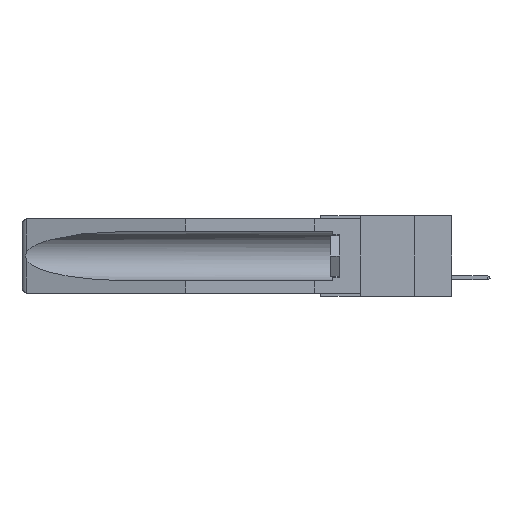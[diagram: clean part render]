
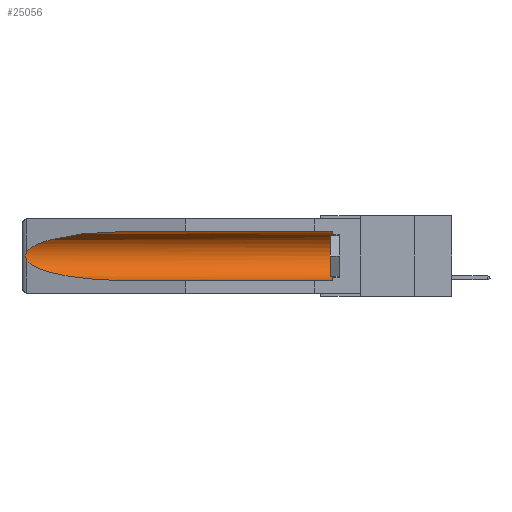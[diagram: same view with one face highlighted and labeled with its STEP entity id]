
A CAD part, left-side view. The second image highlights one B-rep face of the part: STEP entity #25056.
In plain terms, the highlighted cylindrical face has radius 2.857 mm (diameter 5.715 mm), a partial arc.
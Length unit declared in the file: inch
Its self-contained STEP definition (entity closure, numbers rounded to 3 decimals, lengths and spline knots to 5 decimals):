
#21 = CARTESIAN_POINT ( 'NONE',  ( 0.155, 1.07973, -0.284 ) ) ;
#524 = CARTESIAN_POINT ( 'NONE',  ( 0.155, 1.07973, -0.059 ) ) ;
#2341 = DIRECTION ( 'NONE',  ( 0., 1., 0. ) ) ;
#3366 = EDGE_CURVE ( 'NONE', #17460, #10818, #11243, .T. ) ;
#3832 = CIRCLE ( 'NONE', #13570, 0.1125 ) ;
#3856 =( BOUNDED_CURVE ( )  B_SPLINE_CURVE ( 3, ( #12913, #20463, #23338, #21 ),
 .UNSPECIFIED., .F., .F. ) 
 B_SPLINE_CURVE_WITH_KNOTS ( ( 4, 4 ),
 ( 0.1948, 1.5708 ),
 .UNSPECIFIED. ) 
 CURVE ( )  GEOMETRIC_REPRESENTATION_ITEM ( )  RATIONAL_B_SPLINE_CURVE ( ( 1., 0.848, 0.848, 1. ) ) 
 REPRESENTATION_ITEM ( '' )  );
#3952 = DIRECTION ( 'NONE',  ( 0., 1., 0. ) ) ;
#4195 = AXIS2_PLACEMENT_3D ( 'NONE', #27512, #2341, #12525 ) ;
#4275 = ORIENTED_EDGE ( 'NONE', *, *, #18997, .T. ) ;
#5678 = EDGE_CURVE ( 'NONE', #18760, #17460, #15857, .T. ) ;
#6527 = CARTESIAN_POINT ( 'NONE',  ( 0.26597, 1.5296, -0.19026 ) ) ;
#7708 = CARTESIAN_POINT ( 'NONE',  ( 0.26537, 1.52718, -0.19328 ) ) ;
#8341 = CARTESIAN_POINT ( 'NONE',  ( 0.2675, 1.53308, -0.17534 ) ) ;
#8485 = CARTESIAN_POINT ( 'NONE',  ( 0.21114, 1.30732, -0.059 ) ) ;
#9053 = ORIENTED_EDGE ( 'NONE', *, *, #28622, .F. ) ;
#9091 = CARTESIAN_POINT ( 'NONE',  ( 0.26655, 1.53094, -0.18657 ) ) ;
#9796 = CARTESIAN_POINT ( 'NONE',  ( 0.26597, 1.52961, -0.15275 ) ) ;
#10030 = CARTESIAN_POINT ( 'NONE',  ( 0.155, -0.30754, -0.059 ) ) ;
#10818 = VERTEX_POINT ( 'NONE', #28492 ) ;
#11243 =( BOUNDED_CURVE ( )  B_SPLINE_CURVE ( 3, ( #524, #8485, #18940, #16122 ),
 .UNSPECIFIED., .F., .F. ) 
 B_SPLINE_CURVE_WITH_KNOTS ( ( 4, 4 ),
 ( 4.71239, 6.08839 ),
 .UNSPECIFIED. ) 
 CURVE ( )  GEOMETRIC_REPRESENTATION_ITEM ( )  RATIONAL_B_SPLINE_CURVE ( ( 1., 0.848, 0.848, 1. ) ) 
 REPRESENTATION_ITEM ( '' )  );
#12525 = DIRECTION ( 'NONE',  ( 0., 0., 1. ) ) ;
#12913 = CARTESIAN_POINT ( 'NONE',  ( 0.26537, 1.52718, -0.19328 ) ) ;
#13020 = EDGE_CURVE ( 'NONE', #19597, #18760, #3832, .T. ) ;
#13570 = AXIS2_PLACEMENT_3D ( 'NONE', #16858, #19249, #19352 ) ;
#13711 = VERTEX_POINT ( 'NONE', #7708 ) ;
#14286 = VECTOR ( 'NONE', #3952, 39.37008 ) ;
#15514 = CYLINDRICAL_SURFACE ( 'NONE', #4195, 0.1125 ) ;
#15831 = ORIENTED_EDGE ( 'NONE', *, *, #3366, .T. ) ;
#15857 = LINE ( 'NONE', #10030, #21858 ) ;
#16122 = CARTESIAN_POINT ( 'NONE',  ( 0.26537, 1.52718, -0.14972 ) ) ;
#16412 = CARTESIAN_POINT ( 'NONE',  ( 0.26537, 1.52718, -0.19328 ) ) ;
#16858 = CARTESIAN_POINT ( 'NONE',  ( 0.155, 0.126, -0.1715 ) ) ;
#17098 = LINE ( 'NONE', #28050, #14286 ) ;
#17460 = VERTEX_POINT ( 'NONE', #24716 ) ;
#17918 = FACE_OUTER_BOUND ( 'NONE', #21336, .T. ) ;
#18224 = ORIENTED_EDGE ( 'NONE', *, *, #5678, .T. ) ;
#18643 = CARTESIAN_POINT ( 'NONE',  ( 0.155, 0.126, -0.284 ) ) ;
#18760 = VERTEX_POINT ( 'NONE', #28683 ) ;
#18940 = CARTESIAN_POINT ( 'NONE',  ( 0.25451, 1.48313, -0.09465 ) ) ;
#18997 = EDGE_CURVE ( 'NONE', #10818, #13711, #27654, .T. ) ;
#19033 = VERTEX_POINT ( 'NONE', #26247 ) ;
#19249 = DIRECTION ( 'NONE',  ( 0., -1., 0. ) ) ;
#19352 = DIRECTION ( 'NONE',  ( 0., 0., 1. ) ) ;
#19597 = VERTEX_POINT ( 'NONE', #18643 ) ;
#20251 = DIRECTION ( 'NONE',  ( 0., 1., 0. ) ) ;
#20463 = CARTESIAN_POINT ( 'NONE',  ( 0.25451, 1.48313, -0.24835 ) ) ;
#21336 = EDGE_LOOP ( 'NONE', ( #15831, #4275, #31972, #9053, #23360, #18224 ) ) ;
#21858 = VECTOR ( 'NONE', #20251, 39.37008 ) ;
#22178 = EDGE_CURVE ( 'NONE', #13711, #19033, #3856, .T. ) ;
#22583 = CARTESIAN_POINT ( 'NONE',  ( 0.26537, 1.52718, -0.14972 ) ) ;
#23338 = CARTESIAN_POINT ( 'NONE',  ( 0.21114, 1.30732, -0.284 ) ) ;
#23360 = ORIENTED_EDGE ( 'NONE', *, *, #13020, .T. ) ;
#23674 = CARTESIAN_POINT ( 'NONE',  ( 0.26654, 1.53092, -0.15636 ) ) ;
#24716 = CARTESIAN_POINT ( 'NONE',  ( 0.155, 1.07973, -0.059 ) ) ;
#25056 = ADVANCED_FACE ( 'NONE', ( #17918 ), #15514, .F. ) ;
#26247 = CARTESIAN_POINT ( 'NONE',  ( 0.155, 1.07973, -0.284 ) ) ;
#26582 = CARTESIAN_POINT ( 'NONE',  ( 0.2673, 1.5327, -0.16383 ) ) ;
#27512 = CARTESIAN_POINT ( 'NONE',  ( 0.155, -0.30754, -0.1715 ) ) ;
#27654 = B_SPLINE_CURVE_WITH_KNOTS ( 'NONE', 3,
 ( #22583, #9796, #23674, #26582, #29179, #8341, #31775, #9091, #6527, #16412 ),
 .UNSPECIFIED., .F., .F.,
 ( 4, 2, 2, 2, 4 ),
 ( 0., 0.00029, 0.00058, 0.00087, 0.00117 ),
 .UNSPECIFIED. ) ;
#28050 = CARTESIAN_POINT ( 'NONE',  ( 0.155, -0.30754, -0.284 ) ) ;
#28492 = CARTESIAN_POINT ( 'NONE',  ( 0.26537, 1.52718, -0.14972 ) ) ;
#28622 = EDGE_CURVE ( 'NONE', #19597, #19033, #17098, .T. ) ;
#28683 = CARTESIAN_POINT ( 'NONE',  ( 0.155, 0.126, -0.059 ) ) ;
#29179 = CARTESIAN_POINT ( 'NONE',  ( 0.2675, 1.53308, -0.16763 ) ) ;
#31775 = CARTESIAN_POINT ( 'NONE',  ( 0.2673, 1.53269, -0.17917 ) ) ;
#31972 = ORIENTED_EDGE ( 'NONE', *, *, #22178, .T. ) ;
